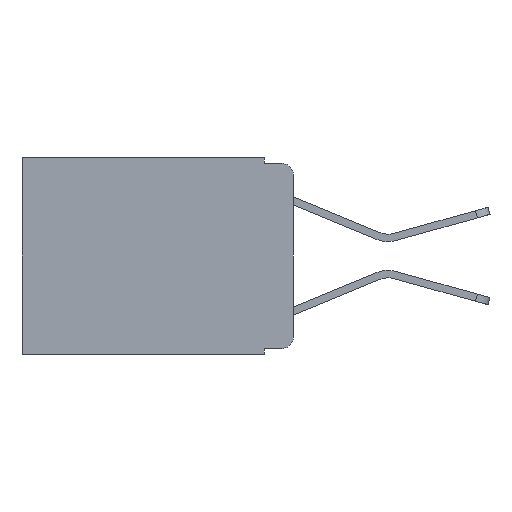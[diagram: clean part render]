
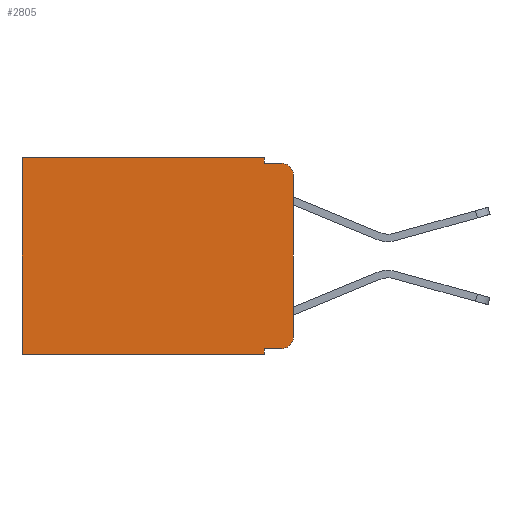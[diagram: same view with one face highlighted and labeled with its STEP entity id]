
A CAD part, left-side view. The second image highlights one B-rep face of the part: STEP entity #2805.
In plain terms, the highlighted planar face has unit normal (-1, 0, 0).
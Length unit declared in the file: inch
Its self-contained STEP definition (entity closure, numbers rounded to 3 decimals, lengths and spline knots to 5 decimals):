
#191 = CARTESIAN_POINT ( 'NONE',  ( 0.298, 0.051, -0.333 ) ) ;
#336 = CARTESIAN_POINT ( 'NONE',  ( 0.298, 0., 0. ) ) ;
#506 = EDGE_CURVE ( 'NONE', #6020, #1336, #4265, .T. ) ;
#737 = EDGE_CURVE ( 'NONE', #3759, #9852, #2658, .T. ) ;
#749 = DIRECTION ( 'NONE',  ( 0., 0., -1. ) ) ;
#800 = ORIENTED_EDGE ( 'NONE', *, *, #1936, .F. ) ;
#1093 = AXIS2_PLACEMENT_3D ( 'NONE', #6897, #2279, #7629 ) ;
#1135 = ORIENTED_EDGE ( 'NONE', *, *, #2290, .F. ) ;
#1251 = CARTESIAN_POINT ( 'NONE',  ( 0.298, 0., -0.313 ) ) ;
#1336 = VERTEX_POINT ( 'NONE', #7845 ) ;
#1559 = CARTESIAN_POINT ( 'NONE',  ( 0.298, 0.051, 0. ) ) ;
#1629 = EDGE_LOOP ( 'NONE', ( #1135, #6194, #8812, #4452, #6094, #7132, #9329, #800, #8359, #6717 ) ) ;
#1647 = VECTOR ( 'NONE', #7174, 39.37008 ) ;
#1738 = CARTESIAN_POINT ( 'NONE',  ( 0.298, 0.051, -0.333 ) ) ;
#1936 = EDGE_CURVE ( 'NONE', #8296, #3759, #9159, .T. ) ;
#2042 = CARTESIAN_POINT ( 'NONE',  ( 0.298, 0.051, 0. ) ) ;
#2103 = LINE ( 'NONE', #336, #9823 ) ;
#2119 = DIRECTION ( 'NONE',  ( -1., 0., 0. ) ) ;
#2279 = DIRECTION ( 'NONE',  ( -1., 0., 0. ) ) ;
#2290 = EDGE_CURVE ( 'NONE', #6020, #7165, #2103, .T. ) ;
#2421 = DIRECTION ( 'NONE',  ( 0., 0., -1. ) ) ;
#2503 = AXIS2_PLACEMENT_3D ( 'NONE', #9062, #8807, #8738 ) ;
#2658 = LINE ( 'NONE', #6377, #5565 ) ;
#2805 = ADVANCED_FACE ( 'NONE', ( #8180 ), #8806, .F. ) ;
#3347 = VECTOR ( 'NONE', #749, 39.37008 ) ;
#3399 = CARTESIAN_POINT ( 'NONE',  ( 0.298, 0.02, -0.03 ) ) ;
#3747 = VECTOR ( 'NONE', #5149, 39.37008 ) ;
#3759 = VERTEX_POINT ( 'NONE', #4356 ) ;
#3832 = LINE ( 'NONE', #1738, #1647 ) ;
#3892 = DIRECTION ( 'NONE',  ( 0., 1., 0. ) ) ;
#4003 = EDGE_CURVE ( 'NONE', #7377, #7009, #9236, .T. ) ;
#4169 = LINE ( 'NONE', #7658, #8127 ) ;
#4178 = LINE ( 'NONE', #6469, #7900 ) ;
#4265 = CIRCLE ( 'NONE', #5122, 0.02 ) ;
#4356 = CARTESIAN_POINT ( 'NONE',  ( 0.298, 0.051, -0.343 ) ) ;
#4452 = ORIENTED_EDGE ( 'NONE', *, *, #4003, .F. ) ;
#4504 = VERTEX_POINT ( 'NONE', #9440 ) ;
#4747 = VERTEX_POINT ( 'NONE', #8077 ) ;
#5109 = CARTESIAN_POINT ( 'NONE',  ( 0.298, 0.051, -0.01 ) ) ;
#5122 = AXIS2_PLACEMENT_3D ( 'NONE', #3399, #2119, #5288 ) ;
#5149 = DIRECTION ( 'NONE',  ( 0., 0., -1. ) ) ;
#5288 = DIRECTION ( 'NONE',  ( 0., 0., -1. ) ) ;
#5391 = CIRCLE ( 'NONE', #1093, 0.02 ) ;
#5540 = VECTOR ( 'NONE', #9657, 39.37008 ) ;
#5565 = VECTOR ( 'NONE', #3892, 39.37008 ) ;
#5604 = CARTESIAN_POINT ( 'NONE',  ( 0.298, 0.051, 0. ) ) ;
#5876 = DIRECTION ( 'NONE',  ( 0., -1., 0. ) ) ;
#6020 = VERTEX_POINT ( 'NONE', #6091 ) ;
#6030 = EDGE_CURVE ( 'NONE', #7009, #1336, #4169, .T. ) ;
#6091 = CARTESIAN_POINT ( 'NONE',  ( 0.298, 0., -0.03 ) ) ;
#6094 = ORIENTED_EDGE ( 'NONE', *, *, #9402, .T. ) ;
#6194 = ORIENTED_EDGE ( 'NONE', *, *, #506, .T. ) ;
#6377 = CARTESIAN_POINT ( 'NONE',  ( 0.298, 0., -0.343 ) ) ;
#6469 = CARTESIAN_POINT ( 'NONE',  ( 0.298, 0., 0. ) ) ;
#6717 = ORIENTED_EDGE ( 'NONE', *, *, #8482, .T. ) ;
#6897 = CARTESIAN_POINT ( 'NONE',  ( 0.298, 0.02, -0.313 ) ) ;
#7009 = VERTEX_POINT ( 'NONE', #5109 ) ;
#7021 = EDGE_CURVE ( 'NONE', #4747, #9852, #7728, .T. ) ;
#7054 = CARTESIAN_POINT ( 'NONE',  ( 0.298, 0.473, -0.343 ) ) ;
#7132 = ORIENTED_EDGE ( 'NONE', *, *, #7021, .T. ) ;
#7165 = VERTEX_POINT ( 'NONE', #1251 ) ;
#7174 = DIRECTION ( 'NONE',  ( 0., -1., 0. ) ) ;
#7377 = VERTEX_POINT ( 'NONE', #1559 ) ;
#7629 = DIRECTION ( 'NONE',  ( 0., 0., -1. ) ) ;
#7658 = CARTESIAN_POINT ( 'NONE',  ( 0.298, 0.051, -0.01 ) ) ;
#7728 = LINE ( 'NONE', #8768, #3747 ) ;
#7845 = CARTESIAN_POINT ( 'NONE',  ( 0.298, 0.02, -0.01 ) ) ;
#7900 = VECTOR ( 'NONE', #10056, 39.37008 ) ;
#8077 = CARTESIAN_POINT ( 'NONE',  ( 0.298, 0.473, 0. ) ) ;
#8127 = VECTOR ( 'NONE', #5876, 39.37008 ) ;
#8180 = FACE_OUTER_BOUND ( 'NONE', #1629, .T. ) ;
#8296 = VERTEX_POINT ( 'NONE', #191 ) ;
#8359 = ORIENTED_EDGE ( 'NONE', *, *, #8848, .T. ) ;
#8482 = EDGE_CURVE ( 'NONE', #4504, #7165, #5391, .T. ) ;
#8738 = DIRECTION ( 'NONE',  ( 0., 0., -1. ) ) ;
#8768 = CARTESIAN_POINT ( 'NONE',  ( 0.298, 0.473, 0. ) ) ;
#8806 = PLANE ( 'NONE',  #2503 ) ;
#8807 = DIRECTION ( 'NONE',  ( 1., 0., 0. ) ) ;
#8812 = ORIENTED_EDGE ( 'NONE', *, *, #6030, .F. ) ;
#8848 = EDGE_CURVE ( 'NONE', #8296, #4504, #3832, .T. ) ;
#9062 = CARTESIAN_POINT ( 'NONE',  ( 0.298, 0., 0. ) ) ;
#9159 = LINE ( 'NONE', #5604, #5540 ) ;
#9236 = LINE ( 'NONE', #2042, #3347 ) ;
#9329 = ORIENTED_EDGE ( 'NONE', *, *, #737, .F. ) ;
#9402 = EDGE_CURVE ( 'NONE', #7377, #4747, #4178, .T. ) ;
#9440 = CARTESIAN_POINT ( 'NONE',  ( 0.298, 0.02, -0.333 ) ) ;
#9657 = DIRECTION ( 'NONE',  ( 0., 0., -1. ) ) ;
#9823 = VECTOR ( 'NONE', #2421, 39.37008 ) ;
#9852 = VERTEX_POINT ( 'NONE', #7054 ) ;
#10056 = DIRECTION ( 'NONE',  ( 0., 1., 0. ) ) ;
